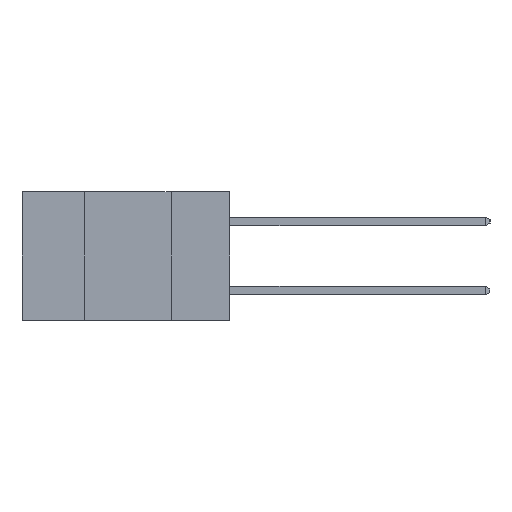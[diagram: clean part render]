
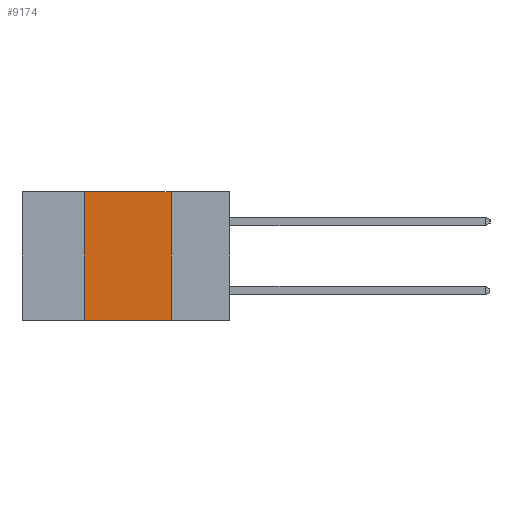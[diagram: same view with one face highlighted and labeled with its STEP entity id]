
A CAD part, left-side view. The second image highlights one B-rep face of the part: STEP entity #9174.
In plain terms, the highlighted planar face has unit normal (-1, 0, 0).
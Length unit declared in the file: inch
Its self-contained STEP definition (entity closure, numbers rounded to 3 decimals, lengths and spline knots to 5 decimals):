
#4 = DIRECTION ( 'NONE',  ( 0., 0., -1. ) ) ;
#216 = DIRECTION ( 'NONE',  ( 0., -1., 0. ) ) ;
#570 = VERTEX_POINT ( 'NONE', #10419 ) ;
#815 = ORIENTED_EDGE ( 'NONE', *, *, #12002, .F. ) ;
#1466 = CARTESIAN_POINT ( 'NONE',  ( 0., 0.6, 0. ) ) ;
#1728 = CARTESIAN_POINT ( 'NONE',  ( 0., 0.42, -0.37 ) ) ;
#1734 = EDGE_LOOP ( 'NONE', ( #4589, #14732, #815, #13084 ) ) ;
#1765 = VERTEX_POINT ( 'NONE', #15206 ) ;
#1882 = CARTESIAN_POINT ( 'NONE',  ( 0., 0.6, -0.37 ) ) ;
#2182 = VERTEX_POINT ( 'NONE', #14254 ) ;
#3226 = CARTESIAN_POINT ( 'NONE',  ( 0., 0.42, 0. ) ) ;
#3844 = VECTOR ( 'NONE', #216, 39.37008 ) ;
#4589 = ORIENTED_EDGE ( 'NONE', *, *, #15120, .F. ) ;
#4619 = VERTEX_POINT ( 'NONE', #1728 ) ;
#4876 = PLANE ( 'NONE',  #5021 ) ;
#5021 = AXIS2_PLACEMENT_3D ( 'NONE', #14659, #7408, #4 ) ;
#5106 = DIRECTION ( 'NONE',  ( 0., 0., -1. ) ) ;
#5533 = VECTOR ( 'NONE', #5106, 39.37008 ) ;
#6259 = VECTOR ( 'NONE', #9325, 39.37008 ) ;
#6670 = LINE ( 'NONE', #3226, #6259 ) ;
#7408 = DIRECTION ( 'NONE',  ( 1., 0., 0. ) ) ;
#8820 = LINE ( 'NONE', #9998, #5533 ) ;
#9174 = ADVANCED_FACE ( 'NONE', ( #11473 ), #4876, .F. ) ;
#9325 = DIRECTION ( 'NONE',  ( 0., 0., 1. ) ) ;
#9998 = CARTESIAN_POINT ( 'NONE',  ( 0., 0.17, 0. ) ) ;
#10419 = CARTESIAN_POINT ( 'NONE',  ( 0., 0.42, 0. ) ) ;
#11473 = FACE_OUTER_BOUND ( 'NONE', #1734, .T. ) ;
#11667 = DIRECTION ( 'NONE',  ( 0., -1., 0. ) ) ;
#11771 = VECTOR ( 'NONE', #11667, 39.37008 ) ;
#12002 = EDGE_CURVE ( 'NONE', #4619, #570, #6670, .T. ) ;
#12855 = EDGE_CURVE ( 'NONE', #4619, #1765, #14958, .T. ) ;
#13084 = ORIENTED_EDGE ( 'NONE', *, *, #12855, .T. ) ;
#13654 = LINE ( 'NONE', #1466, #3844 ) ;
#14254 = CARTESIAN_POINT ( 'NONE',  ( 0., 0.17, 0. ) ) ;
#14274 = EDGE_CURVE ( 'NONE', #570, #2182, #13654, .T. ) ;
#14659 = CARTESIAN_POINT ( 'NONE',  ( 0., 0.6, 0. ) ) ;
#14732 = ORIENTED_EDGE ( 'NONE', *, *, #14274, .F. ) ;
#14958 = LINE ( 'NONE', #1882, #11771 ) ;
#15120 = EDGE_CURVE ( 'NONE', #2182, #1765, #8820, .T. ) ;
#15206 = CARTESIAN_POINT ( 'NONE',  ( 0., 0.17, -0.37 ) ) ;
